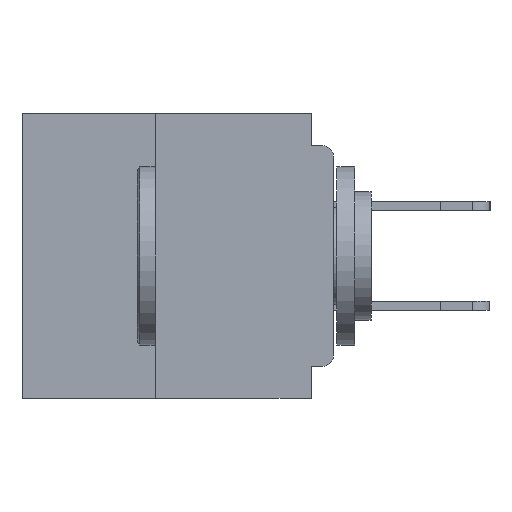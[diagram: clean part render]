
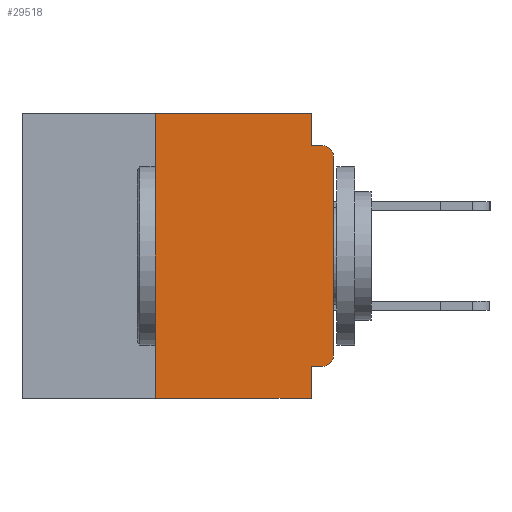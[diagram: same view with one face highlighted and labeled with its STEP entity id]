
A CAD part, left-side view. The second image highlights one B-rep face of the part: STEP entity #29518.
In plain terms, the highlighted planar face has unit normal (-1, 0, 0).
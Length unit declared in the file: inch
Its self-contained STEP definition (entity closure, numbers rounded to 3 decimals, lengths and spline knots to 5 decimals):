
#410 = DIRECTION ( 'NONE',  ( 1., 0., 0. ) ) ;
#576 = VECTOR ( 'NONE', #23308, 39.37008 ) ;
#649 = ORIENTED_EDGE ( 'NONE', *, *, #12688, .F. ) ;
#1224 = AXIS2_PLACEMENT_3D ( 'NONE', #27564, #9069, #30677 ) ;
#1670 = CARTESIAN_POINT ( 'NONE',  ( 0., 0.25, 0. ) ) ;
#2319 = ORIENTED_EDGE ( 'NONE', *, *, #29263, .F. ) ;
#3449 = CARTESIAN_POINT ( 'NONE',  ( 0., 0.031, -0.4 ) ) ;
#3719 = ORIENTED_EDGE ( 'NONE', *, *, #19184, .T. ) ;
#3831 = EDGE_CURVE ( 'NONE', #5251, #36523, #5858, .T. ) ;
#4265 = EDGE_LOOP ( 'NONE', ( #38536, #3719, #33271, #2319, #27510, #37517, #28584, #649, #4708, #35604 ) ) ;
#4708 = ORIENTED_EDGE ( 'NONE', *, *, #31629, .F. ) ;
#4845 = EDGE_CURVE ( 'NONE', #27287, #10072, #34745, .T. ) ;
#5251 = VERTEX_POINT ( 'NONE', #17170 ) ;
#5858 = LINE ( 'NONE', #12839, #30542 ) ;
#5860 = CARTESIAN_POINT ( 'NONE',  ( 0., 0.25, -0.4 ) ) ;
#8772 = CARTESIAN_POINT ( 'NONE',  ( 0., 0.015, -0.06 ) ) ;
#9069 = DIRECTION ( 'NONE',  ( -1., 0., 0. ) ) ;
#9328 = VECTOR ( 'NONE', #12760, 39.37008 ) ;
#9772 = PLANE ( 'NONE',  #38616 ) ;
#10072 = VERTEX_POINT ( 'NONE', #21956 ) ;
#11443 = DIRECTION ( 'NONE',  ( 0., 0., 1. ) ) ;
#11533 = DIRECTION ( 'NONE',  ( 0., 0., -1. ) ) ;
#11541 = CARTESIAN_POINT ( 'NONE',  ( 0., 0.25, -0.4 ) ) ;
#11677 = CARTESIAN_POINT ( 'NONE',  ( 0., 0.031, 0. ) ) ;
#11756 = DIRECTION ( 'NONE',  ( 0., -1., 0. ) ) ;
#11885 = DIRECTION ( 'NONE',  ( 0., 0., -1. ) ) ;
#12688 = EDGE_CURVE ( 'NONE', #18774, #29235, #30987, .T. ) ;
#12760 = DIRECTION ( 'NONE',  ( 0., 1., 0. ) ) ;
#12839 = CARTESIAN_POINT ( 'NONE',  ( 0., 0., -0.045 ) ) ;
#13442 = VERTEX_POINT ( 'NONE', #16182 ) ;
#14019 = CARTESIAN_POINT ( 'NONE',  ( 0., 0., -0.34 ) ) ;
#14413 = CIRCLE ( 'NONE', #1224, 0.015 ) ;
#14529 = VECTOR ( 'NONE', #22083, 39.37008 ) ;
#14779 = LINE ( 'NONE', #11677, #22060 ) ;
#15047 = EDGE_CURVE ( 'NONE', #17676, #32579, #14413, .T. ) ;
#15842 = VECTOR ( 'NONE', #26955, 39.37008 ) ;
#16182 = CARTESIAN_POINT ( 'NONE',  ( 0., 0., -0.06 ) ) ;
#16539 = LINE ( 'NONE', #31274, #9328 ) ;
#16778 = LINE ( 'NONE', #11541, #15842 ) ;
#16789 = EDGE_CURVE ( 'NONE', #33238, #29235, #32596, .T. ) ;
#17170 = CARTESIAN_POINT ( 'NONE',  ( 0., 0.031, -0.045 ) ) ;
#17594 = CARTESIAN_POINT ( 'NONE',  ( 0., 0.031, -0.4 ) ) ;
#17676 = VERTEX_POINT ( 'NONE', #18365 ) ;
#17989 = CIRCLE ( 'NONE', #21700, 0.015 ) ;
#18365 = CARTESIAN_POINT ( 'NONE',  ( 0., 0.015, -0.355 ) ) ;
#18774 = VERTEX_POINT ( 'NONE', #22208 ) ;
#19090 = CARTESIAN_POINT ( 'NONE',  ( 0., 0.437, 0. ) ) ;
#19184 = EDGE_CURVE ( 'NONE', #13442, #36523, #17989, .T. ) ;
#19333 = VECTOR ( 'NONE', #31457, 39.37008 ) ;
#20187 = CARTESIAN_POINT ( 'NONE',  ( 0., 0.437, -0.4 ) ) ;
#21700 = AXIS2_PLACEMENT_3D ( 'NONE', #8772, #30390, #11885 ) ;
#21956 = CARTESIAN_POINT ( 'NONE',  ( 0., 0.031, 0. ) ) ;
#22060 = VECTOR ( 'NONE', #11533, 39.37008 ) ;
#22083 = DIRECTION ( 'NONE',  ( 0., 0., -1. ) ) ;
#22208 = CARTESIAN_POINT ( 'NONE',  ( 0., 0.031, -0.355 ) ) ;
#22222 = DIRECTION ( 'NONE',  ( 0., 0., -1. ) ) ;
#23308 = DIRECTION ( 'NONE',  ( 0., -1., 0. ) ) ;
#25106 = EDGE_CURVE ( 'NONE', #33238, #27287, #16778, .T. ) ;
#26955 = DIRECTION ( 'NONE',  ( 0., 0., 1. ) ) ;
#27287 = VERTEX_POINT ( 'NONE', #1670 ) ;
#27510 = ORIENTED_EDGE ( 'NONE', *, *, #4845, .F. ) ;
#27564 = CARTESIAN_POINT ( 'NONE',  ( 0., 0.015, -0.34 ) ) ;
#28584 = ORIENTED_EDGE ( 'NONE', *, *, #16789, .T. ) ;
#29235 = VERTEX_POINT ( 'NONE', #17594 ) ;
#29263 = EDGE_CURVE ( 'NONE', #10072, #5251, #14779, .T. ) ;
#29518 = ADVANCED_FACE ( 'NONE', ( #29758 ), #9772, .F. ) ;
#29758 = FACE_OUTER_BOUND ( 'NONE', #4265, .T. ) ;
#30390 = DIRECTION ( 'NONE',  ( -1., 0., 0. ) ) ;
#30542 = VECTOR ( 'NONE', #11756, 39.37008 ) ;
#30677 = DIRECTION ( 'NONE',  ( 0., 0., -1. ) ) ;
#30846 = EDGE_CURVE ( 'NONE', #32579, #13442, #36344, .T. ) ;
#30987 = LINE ( 'NONE', #3449, #14529 ) ;
#31274 = CARTESIAN_POINT ( 'NONE',  ( 0., 0., -0.355 ) ) ;
#31457 = DIRECTION ( 'NONE',  ( 0., -1., 0. ) ) ;
#31543 = CARTESIAN_POINT ( 'NONE',  ( 0., 0.437, 0. ) ) ;
#31629 = EDGE_CURVE ( 'NONE', #17676, #18774, #16539, .T. ) ;
#32579 = VERTEX_POINT ( 'NONE', #14019 ) ;
#32596 = LINE ( 'NONE', #20187, #576 ) ;
#33238 = VERTEX_POINT ( 'NONE', #5860 ) ;
#33271 = ORIENTED_EDGE ( 'NONE', *, *, #3831, .F. ) ;
#34745 = LINE ( 'NONE', #31543, #19333 ) ;
#35389 = VECTOR ( 'NONE', #11443, 39.37008 ) ;
#35604 = ORIENTED_EDGE ( 'NONE', *, *, #15047, .T. ) ;
#36344 = LINE ( 'NONE', #38982, #35389 ) ;
#36523 = VERTEX_POINT ( 'NONE', #39646 ) ;
#37517 = ORIENTED_EDGE ( 'NONE', *, *, #25106, .F. ) ;
#38536 = ORIENTED_EDGE ( 'NONE', *, *, #30846, .T. ) ;
#38616 = AXIS2_PLACEMENT_3D ( 'NONE', #19090, #410, #22222 ) ;
#38982 = CARTESIAN_POINT ( 'NONE',  ( 0., 0., 0. ) ) ;
#39646 = CARTESIAN_POINT ( 'NONE',  ( 0., 0.015, -0.045 ) ) ;
